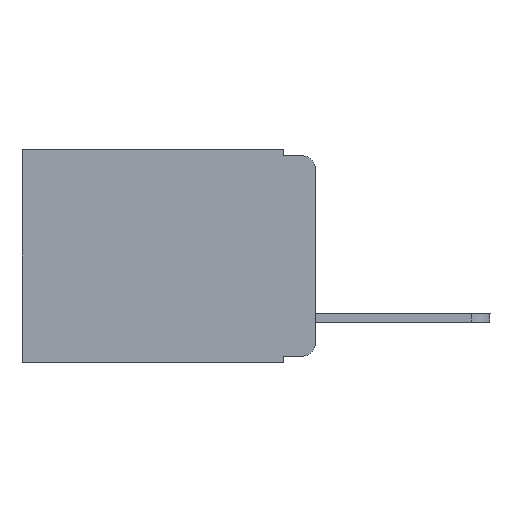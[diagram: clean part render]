
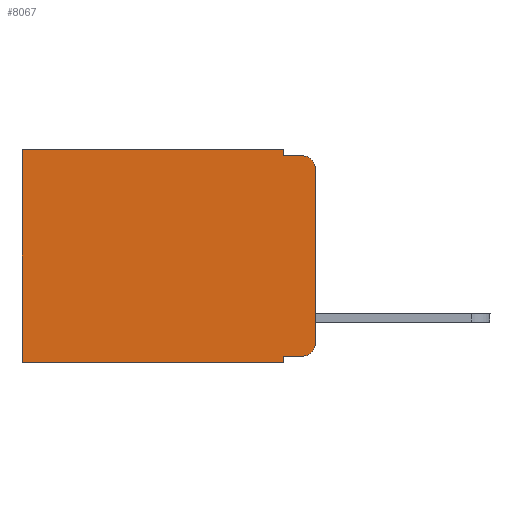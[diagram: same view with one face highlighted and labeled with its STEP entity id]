
A CAD part, left-side view. The second image highlights one B-rep face of the part: STEP entity #8067.
In plain terms, the highlighted planar face has unit normal (-1, 0, 0).
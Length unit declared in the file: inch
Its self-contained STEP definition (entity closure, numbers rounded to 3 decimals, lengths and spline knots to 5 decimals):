
#106 = CARTESIAN_POINT ( 'NONE',  ( 0.298, 0.051, 0. ) ) ;
#451 = CARTESIAN_POINT ( 'NONE',  ( 0.298, 0., -0.03 ) ) ;
#603 = CARTESIAN_POINT ( 'NONE',  ( 0.298, 0.051, -0.333 ) ) ;
#791 = VERTEX_POINT ( 'NONE', #15105 ) ;
#793 = FACE_OUTER_BOUND ( 'NONE', #12310, .T. ) ;
#1008 = CIRCLE ( 'NONE', #16339, 0.02 ) ;
#1168 = ORIENTED_EDGE ( 'NONE', *, *, #4982, .F. ) ;
#1259 = ORIENTED_EDGE ( 'NONE', *, *, #13175, .T. ) ;
#1332 = VERTEX_POINT ( 'NONE', #15160 ) ;
#1639 = DIRECTION ( 'NONE',  ( 0., 0., -1. ) ) ;
#1656 = AXIS2_PLACEMENT_3D ( 'NONE', #5613, #4580, #4500 ) ;
#1760 = DIRECTION ( 'NONE',  ( 0., 0., -1. ) ) ;
#1889 = EDGE_CURVE ( 'NONE', #9525, #9415, #1008, .T. ) ;
#2144 = ORIENTED_EDGE ( 'NONE', *, *, #14624, .F. ) ;
#2558 = ORIENTED_EDGE ( 'NONE', *, *, #1889, .T. ) ;
#2562 = VECTOR ( 'NONE', #6512, 39.37008 ) ;
#2674 = DIRECTION ( 'NONE',  ( 0., -1., 0. ) ) ;
#2919 = VERTEX_POINT ( 'NONE', #12409 ) ;
#2931 = LINE ( 'NONE', #9362, #5416 ) ;
#3310 = EDGE_CURVE ( 'NONE', #7092, #9415, #8186, .T. ) ;
#3392 = LINE ( 'NONE', #9808, #8227 ) ;
#3432 = VERTEX_POINT ( 'NONE', #13963 ) ;
#4141 = EDGE_CURVE ( 'NONE', #8608, #14761, #10853, .T. ) ;
#4171 = DIRECTION ( 'NONE',  ( 0., 0., -1. ) ) ;
#4381 = CARTESIAN_POINT ( 'NONE',  ( 0.298, 0.02, -0.03 ) ) ;
#4500 = DIRECTION ( 'NONE',  ( 0., 0., -1. ) ) ;
#4580 = DIRECTION ( 'NONE',  ( -1., 0., 0. ) ) ;
#4831 = CARTESIAN_POINT ( 'NONE',  ( 0.298, 0., 0. ) ) ;
#4982 = EDGE_CURVE ( 'NONE', #1332, #7092, #2931, .T. ) ;
#5275 = DIRECTION ( 'NONE',  ( 0., 0., -1. ) ) ;
#5288 = ORIENTED_EDGE ( 'NONE', *, *, #15691, .T. ) ;
#5416 = VECTOR ( 'NONE', #7077, 39.37008 ) ;
#5613 = CARTESIAN_POINT ( 'NONE',  ( 0.298, 0.02, -0.313 ) ) ;
#5955 = EDGE_CURVE ( 'NONE', #9525, #791, #11339, .T. ) ;
#5967 = PLANE ( 'NONE',  #8130 ) ;
#6255 = VECTOR ( 'NONE', #5275, 39.37008 ) ;
#6512 = DIRECTION ( 'NONE',  ( 0., 1., 0. ) ) ;
#6557 = ORIENTED_EDGE ( 'NONE', *, *, #8263, .T. ) ;
#6661 = VECTOR ( 'NONE', #7526, 39.37008 ) ;
#6797 = CARTESIAN_POINT ( 'NONE',  ( 0.298, 0.051, -0.01 ) ) ;
#7077 = DIRECTION ( 'NONE',  ( 0., 0., -1. ) ) ;
#7090 = CARTESIAN_POINT ( 'NONE',  ( 0.298, 0.473, -0.343 ) ) ;
#7092 = VERTEX_POINT ( 'NONE', #6797 ) ;
#7296 = VECTOR ( 'NONE', #11262, 39.37008 ) ;
#7526 = DIRECTION ( 'NONE',  ( 0., 1., 0. ) ) ;
#7779 = CARTESIAN_POINT ( 'NONE',  ( 0.298, 0.473, 0. ) ) ;
#8059 = LINE ( 'NONE', #106, #6255 ) ;
#8067 = ADVANCED_FACE ( 'NONE', ( #793 ), #5967, .F. ) ;
#8130 = AXIS2_PLACEMENT_3D ( 'NONE', #16191, #9845, #4171 ) ;
#8186 = LINE ( 'NONE', #13311, #11892 ) ;
#8227 = VECTOR ( 'NONE', #2674, 39.37008 ) ;
#8263 = EDGE_CURVE ( 'NONE', #3432, #791, #11898, .T. ) ;
#8537 = ORIENTED_EDGE ( 'NONE', *, *, #4141, .T. ) ;
#8608 = VERTEX_POINT ( 'NONE', #7779 ) ;
#9325 = CARTESIAN_POINT ( 'NONE',  ( 0.298, 0.02, -0.01 ) ) ;
#9362 = CARTESIAN_POINT ( 'NONE',  ( 0.298, 0.051, 0. ) ) ;
#9415 = VERTEX_POINT ( 'NONE', #9325 ) ;
#9430 = EDGE_CURVE ( 'NONE', #14386, #2919, #8059, .T. ) ;
#9525 = VERTEX_POINT ( 'NONE', #451 ) ;
#9808 = CARTESIAN_POINT ( 'NONE',  ( 0.298, 0.051, -0.333 ) ) ;
#9845 = DIRECTION ( 'NONE',  ( 1., 0., 0. ) ) ;
#10296 = CARTESIAN_POINT ( 'NONE',  ( 0.298, 0., -0.343 ) ) ;
#10301 = CARTESIAN_POINT ( 'NONE',  ( 0.298, 0., 0. ) ) ;
#10466 = LINE ( 'NONE', #10296, #2562 ) ;
#10806 = DIRECTION ( 'NONE',  ( 0., -1., 0. ) ) ;
#10853 = LINE ( 'NONE', #13265, #12187 ) ;
#11262 = DIRECTION ( 'NONE',  ( 0., 0., -1. ) ) ;
#11313 = ORIENTED_EDGE ( 'NONE', *, *, #3310, .F. ) ;
#11339 = LINE ( 'NONE', #4831, #7296 ) ;
#11806 = ORIENTED_EDGE ( 'NONE', *, *, #5955, .F. ) ;
#11892 = VECTOR ( 'NONE', #10806, 39.37008 ) ;
#11898 = CIRCLE ( 'NONE', #1656, 0.02 ) ;
#12187 = VECTOR ( 'NONE', #1639, 39.37008 ) ;
#12310 = EDGE_LOOP ( 'NONE', ( #11806, #2558, #11313, #1168, #5288, #8537, #2144, #12907, #1259, #6557 ) ) ;
#12409 = CARTESIAN_POINT ( 'NONE',  ( 0.298, 0.051, -0.343 ) ) ;
#12731 = LINE ( 'NONE', #10301, #6661 ) ;
#12907 = ORIENTED_EDGE ( 'NONE', *, *, #9430, .F. ) ;
#13175 = EDGE_CURVE ( 'NONE', #14386, #3432, #3392, .T. ) ;
#13265 = CARTESIAN_POINT ( 'NONE',  ( 0.298, 0.473, 0. ) ) ;
#13311 = CARTESIAN_POINT ( 'NONE',  ( 0.298, 0.051, -0.01 ) ) ;
#13963 = CARTESIAN_POINT ( 'NONE',  ( 0.298, 0.02, -0.333 ) ) ;
#14386 = VERTEX_POINT ( 'NONE', #603 ) ;
#14624 = EDGE_CURVE ( 'NONE', #2919, #14761, #10466, .T. ) ;
#14761 = VERTEX_POINT ( 'NONE', #7090 ) ;
#15105 = CARTESIAN_POINT ( 'NONE',  ( 0.298, 0., -0.313 ) ) ;
#15160 = CARTESIAN_POINT ( 'NONE',  ( 0.298, 0.051, 0. ) ) ;
#15691 = EDGE_CURVE ( 'NONE', #1332, #8608, #12731, .T. ) ;
#15702 = DIRECTION ( 'NONE',  ( -1., 0., 0. ) ) ;
#16191 = CARTESIAN_POINT ( 'NONE',  ( 0.298, 0., 0. ) ) ;
#16339 = AXIS2_PLACEMENT_3D ( 'NONE', #4381, #15702, #1760 ) ;
